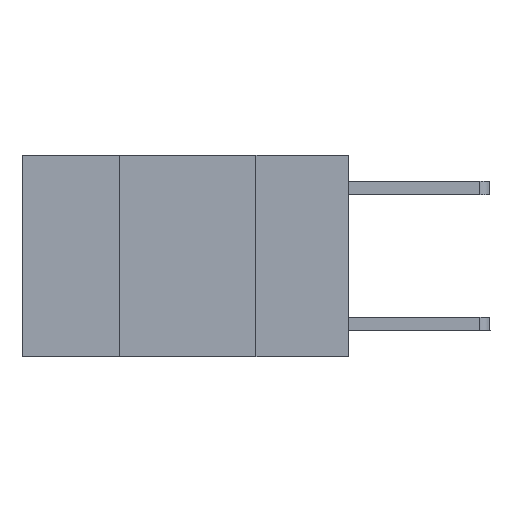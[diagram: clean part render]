
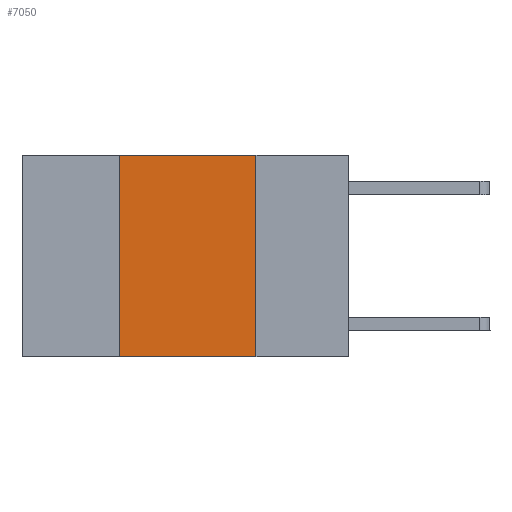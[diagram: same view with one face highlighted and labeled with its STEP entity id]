
A CAD part, left-side view. The second image highlights one B-rep face of the part: STEP entity #7050.
In plain terms, the highlighted planar face has unit normal (-1, 0, 0).
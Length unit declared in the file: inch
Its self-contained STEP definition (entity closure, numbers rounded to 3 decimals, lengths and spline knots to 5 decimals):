
#188 = ORIENTED_EDGE ( 'NONE', *, *, #9122, .F. ) ;
#385 = CARTESIAN_POINT ( 'NONE',  ( 0., 0.6, 0. ) ) ;
#568 = CARTESIAN_POINT ( 'NONE',  ( 0., 0.17, 0. ) ) ;
#1313 = VECTOR ( 'NONE', #5779, 39.37008 ) ;
#1578 = DIRECTION ( 'NONE',  ( 0., 0., -1. ) ) ;
#1627 = DIRECTION ( 'NONE',  ( 0., -1., 0. ) ) ;
#1659 = CARTESIAN_POINT ( 'NONE',  ( 0., 0.42, 0. ) ) ;
#2399 = VERTEX_POINT ( 'NONE', #1659 ) ;
#2578 = DIRECTION ( 'NONE',  ( 0., 0., 1. ) ) ;
#3343 = LINE ( 'NONE', #11764, #1313 ) ;
#4445 = DIRECTION ( 'NONE',  ( 1., 0., 0. ) ) ;
#4664 = VECTOR ( 'NONE', #1627, 39.37008 ) ;
#4930 = VERTEX_POINT ( 'NONE', #10044 ) ;
#5625 = EDGE_LOOP ( 'NONE', ( #188, #8598, #11037, #10627 ) ) ;
#5779 = DIRECTION ( 'NONE',  ( 0., -1., 0. ) ) ;
#6369 = PLANE ( 'NONE',  #8475 ) ;
#7050 = ADVANCED_FACE ( 'NONE', ( #8210 ), #6369, .F. ) ;
#7860 = EDGE_CURVE ( 'NONE', #2399, #4930, #3343, .T. ) ;
#8105 = LINE ( 'NONE', #568, #11913 ) ;
#8210 = FACE_OUTER_BOUND ( 'NONE', #5625, .T. ) ;
#8446 = CARTESIAN_POINT ( 'NONE',  ( 0., 0.6, -0.37 ) ) ;
#8475 = AXIS2_PLACEMENT_3D ( 'NONE', #385, #4445, #10769 ) ;
#8598 = ORIENTED_EDGE ( 'NONE', *, *, #7860, .F. ) ;
#9122 = EDGE_CURVE ( 'NONE', #4930, #10577, #8105, .T. ) ;
#9140 = EDGE_CURVE ( 'NONE', #11758, #2399, #9905, .T. ) ;
#9153 = EDGE_CURVE ( 'NONE', #11758, #10577, #11456, .T. ) ;
#9905 = LINE ( 'NONE', #10145, #11680 ) ;
#10044 = CARTESIAN_POINT ( 'NONE',  ( 0., 0.17, 0. ) ) ;
#10145 = CARTESIAN_POINT ( 'NONE',  ( 0., 0.42, 0. ) ) ;
#10577 = VERTEX_POINT ( 'NONE', #11192 ) ;
#10627 = ORIENTED_EDGE ( 'NONE', *, *, #9153, .T. ) ;
#10769 = DIRECTION ( 'NONE',  ( 0., 0., -1. ) ) ;
#11037 = ORIENTED_EDGE ( 'NONE', *, *, #9140, .F. ) ;
#11192 = CARTESIAN_POINT ( 'NONE',  ( 0., 0.17, -0.37 ) ) ;
#11456 = LINE ( 'NONE', #8446, #4664 ) ;
#11556 = CARTESIAN_POINT ( 'NONE',  ( 0., 0.42, -0.37 ) ) ;
#11680 = VECTOR ( 'NONE', #2578, 39.37008 ) ;
#11758 = VERTEX_POINT ( 'NONE', #11556 ) ;
#11764 = CARTESIAN_POINT ( 'NONE',  ( 0., 0.6, 0. ) ) ;
#11913 = VECTOR ( 'NONE', #1578, 39.37008 ) ;
